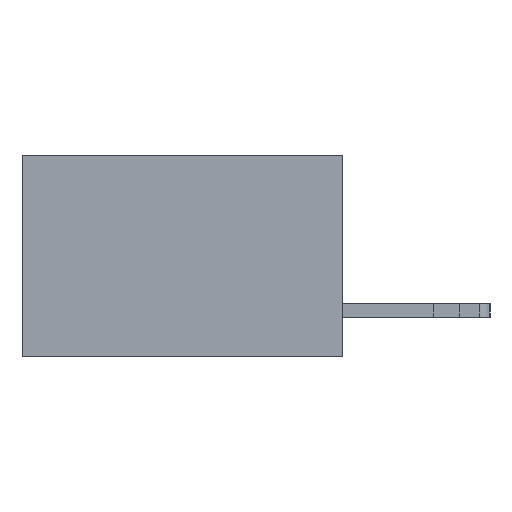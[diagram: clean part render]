
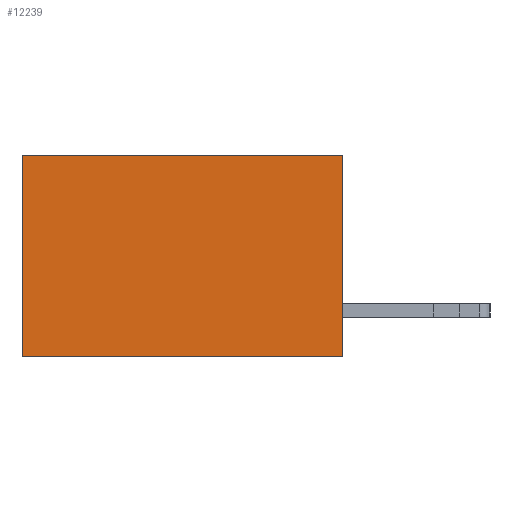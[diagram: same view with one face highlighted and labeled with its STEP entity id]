
A CAD part, left-side view. The second image highlights one B-rep face of the part: STEP entity #12239.
In plain terms, the highlighted planar face has unit normal (-1, 0, 0).
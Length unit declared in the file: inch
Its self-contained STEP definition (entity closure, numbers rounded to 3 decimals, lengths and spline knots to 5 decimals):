
#434 = PLANE ( 'NONE',  #6539 ) ;
#699 = VERTEX_POINT ( 'NONE', #2564 ) ;
#1597 = VERTEX_POINT ( 'NONE', #14391 ) ;
#1859 = VECTOR ( 'NONE', #1996, 39.37008 ) ;
#1870 = ORIENTED_EDGE ( 'NONE', *, *, #7744, .F. ) ;
#1996 = DIRECTION ( 'NONE',  ( 0., 1., 0. ) ) ;
#2564 = CARTESIAN_POINT ( 'NONE',  ( 0.277, 0.59, 0. ) ) ;
#2594 = CARTESIAN_POINT ( 'NONE',  ( 0.277, 0., 0. ) ) ;
#4471 = CARTESIAN_POINT ( 'NONE',  ( 0.277, 0., 0. ) ) ;
#4718 = DIRECTION ( 'NONE',  ( 0., 0., -1. ) ) ;
#4913 = VERTEX_POINT ( 'NONE', #6623 ) ;
#5267 = EDGE_CURVE ( 'NONE', #13262, #699, #11316, .T. ) ;
#5755 = DIRECTION ( 'NONE',  ( 0., 0., -1. ) ) ;
#5874 = LINE ( 'NONE', #7165, #11429 ) ;
#6198 = CARTESIAN_POINT ( 'NONE',  ( 0.277, 0., -0.37 ) ) ;
#6200 = DIRECTION ( 'NONE',  ( 0., 1., 0. ) ) ;
#6539 = AXIS2_PLACEMENT_3D ( 'NONE', #9140, #12338, #5755 ) ;
#6623 = CARTESIAN_POINT ( 'NONE',  ( 0.277, 0.59, -0.37 ) ) ;
#6732 = VECTOR ( 'NONE', #8249, 39.37008 ) ;
#7165 = CARTESIAN_POINT ( 'NONE',  ( 0.277, 0., -0.37 ) ) ;
#7744 = EDGE_CURVE ( 'NONE', #1597, #4913, #13572, .T. ) ;
#7836 = VECTOR ( 'NONE', #6200, 39.37008 ) ;
#8249 = DIRECTION ( 'NONE',  ( 0., 0., -1. ) ) ;
#8337 = EDGE_CURVE ( 'NONE', #13262, #1597, #5874, .T. ) ;
#8881 = EDGE_LOOP ( 'NONE', ( #13442, #1870, #11979, #14752 ) ) ;
#9140 = CARTESIAN_POINT ( 'NONE',  ( 0.277, 0., -0.37 ) ) ;
#9206 = FACE_OUTER_BOUND ( 'NONE', #8881, .T. ) ;
#10581 = EDGE_CURVE ( 'NONE', #699, #4913, #12218, .T. ) ;
#11316 = LINE ( 'NONE', #2594, #1859 ) ;
#11429 = VECTOR ( 'NONE', #4718, 39.37008 ) ;
#11979 = ORIENTED_EDGE ( 'NONE', *, *, #8337, .F. ) ;
#12218 = LINE ( 'NONE', #12578, #6732 ) ;
#12239 = ADVANCED_FACE ( 'NONE', ( #9206 ), #434, .F. ) ;
#12338 = DIRECTION ( 'NONE',  ( 1., 0., 0. ) ) ;
#12578 = CARTESIAN_POINT ( 'NONE',  ( 0.277, 0.59, -0.37 ) ) ;
#13262 = VERTEX_POINT ( 'NONE', #4471 ) ;
#13442 = ORIENTED_EDGE ( 'NONE', *, *, #10581, .T. ) ;
#13572 = LINE ( 'NONE', #6198, #7836 ) ;
#14391 = CARTESIAN_POINT ( 'NONE',  ( 0.277, 0., -0.37 ) ) ;
#14752 = ORIENTED_EDGE ( 'NONE', *, *, #5267, .T. ) ;
